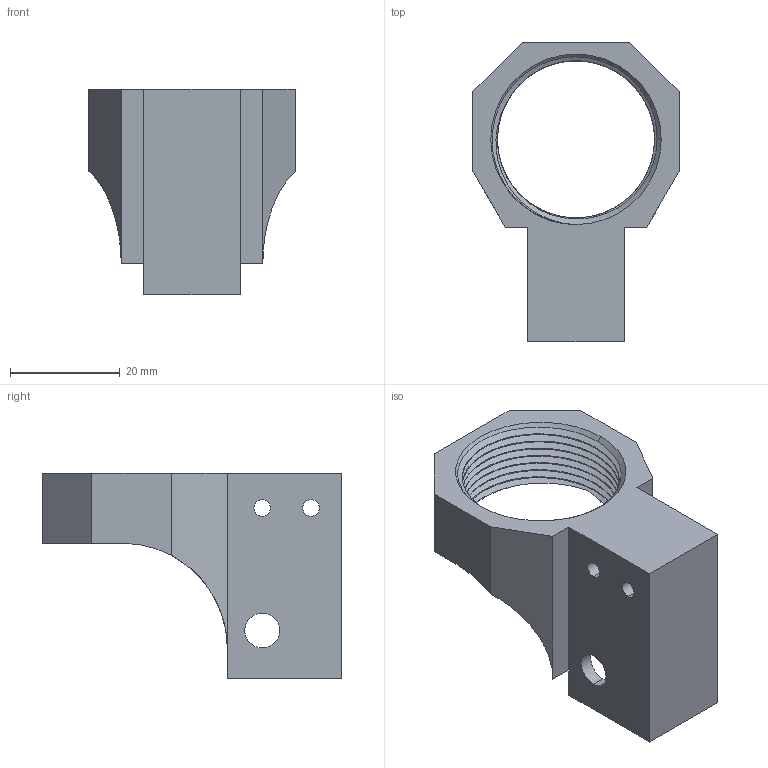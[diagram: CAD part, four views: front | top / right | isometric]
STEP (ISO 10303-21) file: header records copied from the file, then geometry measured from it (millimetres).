
FILE_DESCRIPTION (( 'STEP AP214' ), '1' );
FILE_NAME ('Reinforced_Buffer_Millable.step', '2015-06-12T17:40:45', ( '' ), ( '' ), 'SwSTEP 2.0', 'SolidWorks 2015', '' );
FILE_SCHEMA (( 'AUTOMOTIVE_DESIGN' ));
Length unit declared in the file: millimetre
Products named in the file (1): Reinforced_Buffer_Millable
Bounding box: 37.49 x 54.46 x 37.47 mm (x, y, z)
Volume: 16215.5 mm3; surface area: 9592.5 mm2
Topology: 1 solids, 1 shells, 92 faces, 266 edges, 175 vertices
Faces by surface type: cylinder 37, bspline 27, plane 22, cone 6
Entity records: 26687 total; most frequent: CARTESIAN_POINT 24631, ORIENTED_EDGE 532, DIRECTION 279, EDGE_CURVE 266, VERTEX_POINT 175, B_SPLINE_CURVE_WITH_KNOTS 111, EDGE_LOOP 101, AXIS2_PLACEMENT_3D 98
